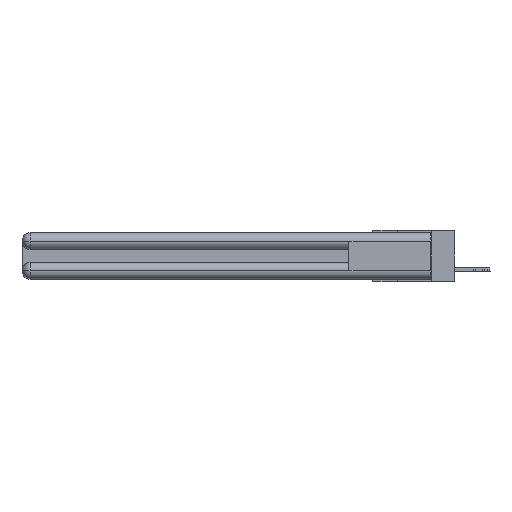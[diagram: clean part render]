
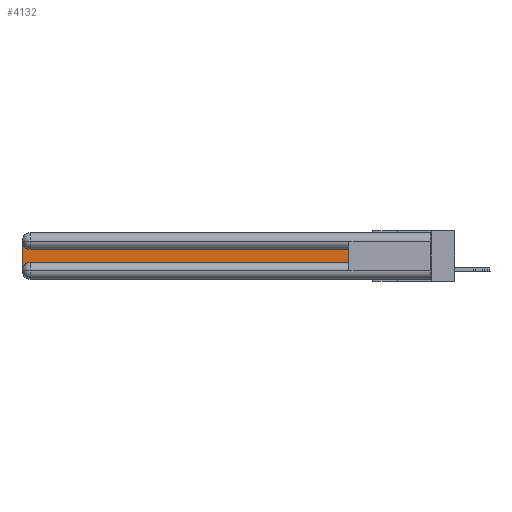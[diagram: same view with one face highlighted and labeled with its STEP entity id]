
A CAD part, left-side view. The second image highlights one B-rep face of the part: STEP entity #4132.
In plain terms, the highlighted planar face has unit normal (-1, 0, 0).
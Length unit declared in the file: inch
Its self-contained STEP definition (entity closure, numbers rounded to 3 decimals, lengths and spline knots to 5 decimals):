
#102 = CARTESIAN_POINT ( 'NONE',  ( 0.075, 3., -0.0625 ) ) ;
#732 = VECTOR ( 'NONE', #3094, 39.37008 ) ;
#863 = ORIENTED_EDGE ( 'NONE', *, *, #25390, .T. ) ;
#1190 = VECTOR ( 'NONE', #26482, 39.37008 ) ;
#1463 = LINE ( 'NONE', #22157, #732 ) ;
#1511 = VERTEX_POINT ( 'NONE', #17238 ) ;
#1938 = LINE ( 'NONE', #3179, #1190 ) ;
#2222 = LINE ( 'NONE', #4732, #26034 ) ;
#2292 = AXIS2_PLACEMENT_3D ( 'NONE', #4757, #14338, #7199 ) ;
#3094 = DIRECTION ( 'NONE',  ( 0., 0., 1. ) ) ;
#3179 = CARTESIAN_POINT ( 'NONE',  ( 0.075, 0.6, -0.2175 ) ) ;
#3698 = ORIENTED_EDGE ( 'NONE', *, *, #21496, .T. ) ;
#4132 = ADVANCED_FACE ( 'NONE', ( #28631 ), #23654, .F. ) ;
#4524 = AXIS2_PLACEMENT_3D ( 'NONE', #18409, #16039, #27949 ) ;
#4709 = VECTOR ( 'NONE', #18801, 39.37008 ) ;
#4732 = CARTESIAN_POINT ( 'NONE',  ( 0.075, 0.6, -0.1225 ) ) ;
#4757 = CARTESIAN_POINT ( 'NONE',  ( 0.075, 3., -0.1225 ) ) ;
#4970 = CARTESIAN_POINT ( 'NONE',  ( 0.075, 2.94, -0.1225 ) ) ;
#5415 = AXIS2_PLACEMENT_3D ( 'NONE', #18838, #21340, #9228 ) ;
#5741 = EDGE_CURVE ( 'NONE', #9484, #5993, #13647, .T. ) ;
#5993 = VERTEX_POINT ( 'NONE', #22102 ) ;
#6952 = CIRCLE ( 'NONE', #4524, 0.06 ) ;
#7199 = DIRECTION ( 'NONE',  ( 0., 0., -1. ) ) ;
#9228 = DIRECTION ( 'NONE',  ( 0., 0., -1. ) ) ;
#9484 = VERTEX_POINT ( 'NONE', #102 ) ;
#9917 = ORIENTED_EDGE ( 'NONE', *, *, #5741, .T. ) ;
#10013 = ORIENTED_EDGE ( 'NONE', *, *, #25989, .T. ) ;
#10629 = EDGE_CURVE ( 'NONE', #28953, #1511, #1463, .T. ) ;
#13647 = LINE ( 'NONE', #26130, #4709 ) ;
#13966 = CARTESIAN_POINT ( 'NONE',  ( 0.075, 2.94, -0.2175 ) ) ;
#14260 = EDGE_CURVE ( 'NONE', #5993, #14830, #6952, .T. ) ;
#14338 = DIRECTION ( 'NONE',  ( 1., 0., 0. ) ) ;
#14830 = VERTEX_POINT ( 'NONE', #13966 ) ;
#16039 = DIRECTION ( 'NONE',  ( 1., 0., 0. ) ) ;
#16354 = ORIENTED_EDGE ( 'NONE', *, *, #10629, .T. ) ;
#17015 = CIRCLE ( 'NONE', #5415, 0.06 ) ;
#17238 = CARTESIAN_POINT ( 'NONE',  ( 0.075, 0.6, -0.1225 ) ) ;
#18409 = CARTESIAN_POINT ( 'NONE',  ( 0.075, 2.94, -0.2775 ) ) ;
#18801 = DIRECTION ( 'NONE',  ( 0., 0., -1. ) ) ;
#18838 = CARTESIAN_POINT ( 'NONE',  ( 0.075, 2.94, -0.0625 ) ) ;
#21340 = DIRECTION ( 'NONE',  ( 1., 0., 0. ) ) ;
#21496 = EDGE_CURVE ( 'NONE', #27131, #9484, #17015, .T. ) ;
#21764 = CARTESIAN_POINT ( 'NONE',  ( 0.075, 0.6, -0.2175 ) ) ;
#22102 = CARTESIAN_POINT ( 'NONE',  ( 0.075, 3., -0.2775 ) ) ;
#22157 = CARTESIAN_POINT ( 'NONE',  ( 0.075, 0.6, -0.2175 ) ) ;
#23113 = DIRECTION ( 'NONE',  ( 0., 1., 0. ) ) ;
#23654 = PLANE ( 'NONE',  #2292 ) ;
#24110 = EDGE_LOOP ( 'NONE', ( #10013, #3698, #9917, #25230, #863, #16354 ) ) ;
#25230 = ORIENTED_EDGE ( 'NONE', *, *, #14260, .T. ) ;
#25390 = EDGE_CURVE ( 'NONE', #14830, #28953, #1938, .T. ) ;
#25989 = EDGE_CURVE ( 'NONE', #1511, #27131, #2222, .T. ) ;
#26034 = VECTOR ( 'NONE', #23113, 39.37008 ) ;
#26130 = CARTESIAN_POINT ( 'NONE',  ( 0.075, 3., -0.2175 ) ) ;
#26482 = DIRECTION ( 'NONE',  ( 0., -1., 0. ) ) ;
#27131 = VERTEX_POINT ( 'NONE', #4970 ) ;
#27949 = DIRECTION ( 'NONE',  ( 0., 0., -1. ) ) ;
#28631 = FACE_OUTER_BOUND ( 'NONE', #24110, .T. ) ;
#28953 = VERTEX_POINT ( 'NONE', #21764 ) ;
